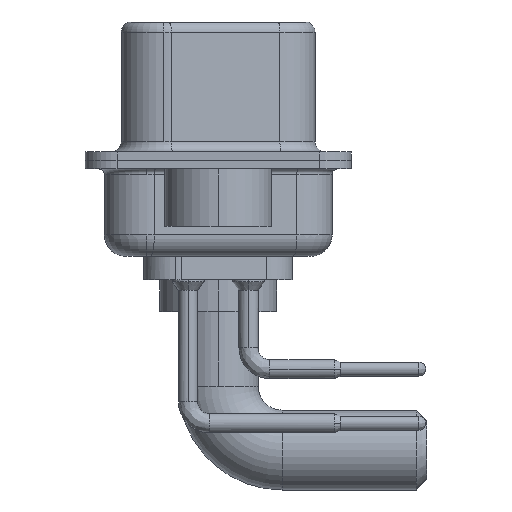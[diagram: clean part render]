
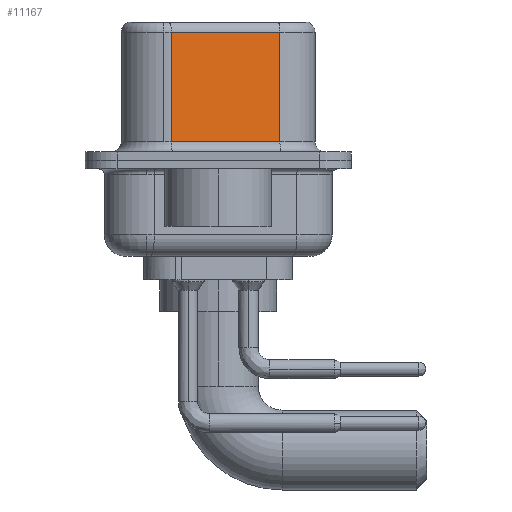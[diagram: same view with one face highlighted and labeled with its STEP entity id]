
A CAD part, left-side view. The second image highlights one B-rep face of the part: STEP entity #11167.
In plain terms, the highlighted planar face has unit normal (-0.985, -0.174, 0).
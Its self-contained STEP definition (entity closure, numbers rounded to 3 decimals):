
#878 = VECTOR ( 'NONE', #13736, 1000. ) ;
#1543 = LINE ( 'NONE', #21597, #878 ) ;
#2616 = ORIENTED_EDGE ( 'NONE', *, *, #15974, .F. ) ;
#2887 = CARTESIAN_POINT ( 'NONE',  ( 4.58, -2.897, 6.52 ) ) ;
#3415 = VECTOR ( 'NONE', #8003, 1000. ) ;
#3432 = AXIS2_PLACEMENT_3D ( 'NONE', #2887, #18870, #12972 ) ;
#4203 = EDGE_LOOP ( 'NONE', ( #2616, #19615, #20680, #7572 ) ) ;
#4442 = LINE ( 'NONE', #20304, #3415 ) ;
#4982 = FACE_OUTER_BOUND ( 'NONE', #4203, .T. ) ;
#5083 = VERTEX_POINT ( 'NONE', #18653 ) ;
#6420 = DIRECTION ( 'NONE',  ( -0.174, 0.985, 0. ) ) ;
#7572 = ORIENTED_EDGE ( 'NONE', *, *, #18034, .T. ) ;
#7735 = VECTOR ( 'NONE', #6420, 1000. ) ;
#7745 = VERTEX_POINT ( 'NONE', #18018 ) ;
#8003 = DIRECTION ( 'NONE',  ( 0.174, -0.985, 0. ) ) ;
#11167 = ADVANCED_FACE ( 'NONE', ( #4982 ), #12851, .F. ) ;
#11375 = VERTEX_POINT ( 'NONE', #16438 ) ;
#12851 = PLANE ( 'NONE',  #3432 ) ;
#12972 = DIRECTION ( 'NONE',  ( -0.174, 0.985, 0. ) ) ;
#13736 = DIRECTION ( 'NONE',  ( 0., 0., -1. ) ) ;
#14150 = CARTESIAN_POINT ( 'NONE',  ( 3.68, 2.203, 6.52 ) ) ;
#15974 = EDGE_CURVE ( 'NONE', #11375, #5083, #1543, .T. ) ;
#16438 = CARTESIAN_POINT ( 'NONE',  ( 4.58, -2.897, 6.02 ) ) ;
#18018 = CARTESIAN_POINT ( 'NONE',  ( 3.68, 2.203, 0.9 ) ) ;
#18034 = EDGE_CURVE ( 'NONE', #7745, #5083, #4442, .T. ) ;
#18653 = CARTESIAN_POINT ( 'NONE',  ( 4.58, -2.897, 0.9 ) ) ;
#18870 = DIRECTION ( 'NONE',  ( 0.985, 0.174, 0. ) ) ;
#18979 = VERTEX_POINT ( 'NONE', #22295 ) ;
#19425 = EDGE_CURVE ( 'NONE', #18979, #7745, #20308, .T. ) ;
#19615 = ORIENTED_EDGE ( 'NONE', *, *, #21036, .T. ) ;
#19771 = VECTOR ( 'NONE', #22147, 1000. ) ;
#20304 = CARTESIAN_POINT ( 'NONE',  ( 4.58, -2.897, 0.9 ) ) ;
#20308 = LINE ( 'NONE', #14150, #19771 ) ;
#20680 = ORIENTED_EDGE ( 'NONE', *, *, #19425, .T. ) ;
#20833 = CARTESIAN_POINT ( 'NONE',  ( 4.58, -2.897, 6.02 ) ) ;
#21036 = EDGE_CURVE ( 'NONE', #11375, #18979, #24379, .T. ) ;
#21597 = CARTESIAN_POINT ( 'NONE',  ( 4.58, -2.897, 6.52 ) ) ;
#22147 = DIRECTION ( 'NONE',  ( 0., 0., -1. ) ) ;
#22295 = CARTESIAN_POINT ( 'NONE',  ( 3.68, 2.203, 6.02 ) ) ;
#24379 = LINE ( 'NONE', #20833, #7735 ) ;
